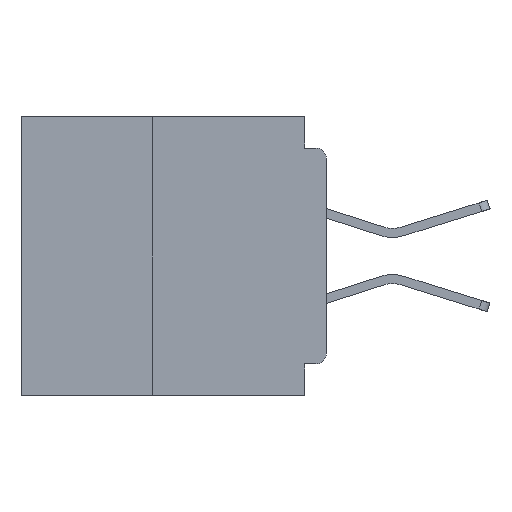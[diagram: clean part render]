
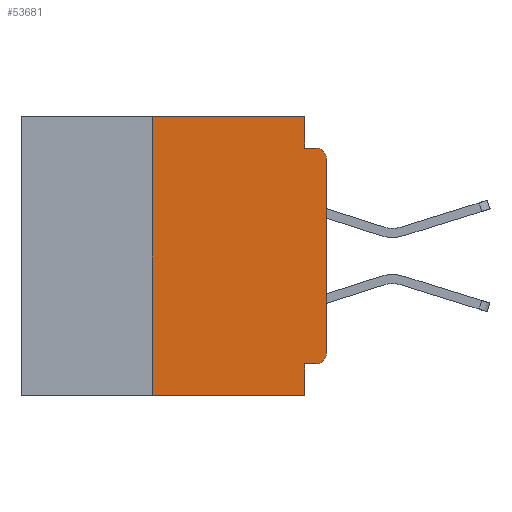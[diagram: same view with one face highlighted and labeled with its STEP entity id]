
A CAD part, left-side view. The second image highlights one B-rep face of the part: STEP entity #53681.
In plain terms, the highlighted planar face has unit normal (-1, 0, 0).
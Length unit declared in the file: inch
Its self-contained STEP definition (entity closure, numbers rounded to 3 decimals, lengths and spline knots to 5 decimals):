
#747 = ORIENTED_EDGE ( 'NONE', *, *, #26089, .T. ) ;
#2071 = CIRCLE ( 'NONE', #11565, 0.015 ) ;
#2143 = ORIENTED_EDGE ( 'NONE', *, *, #19989, .F. ) ;
#2310 = EDGE_CURVE ( 'NONE', #57556, #36472, #18998, .T. ) ;
#2334 = CARTESIAN_POINT ( 'NONE',  ( 0., 0., -0.06 ) ) ;
#3139 = CARTESIAN_POINT ( 'NONE',  ( 0., 0.015, -0.34 ) ) ;
#3239 = VERTEX_POINT ( 'NONE', #44509 ) ;
#3840 = CARTESIAN_POINT ( 'NONE',  ( 0., 0., -0.355 ) ) ;
#3991 = VERTEX_POINT ( 'NONE', #36102 ) ;
#4063 = CARTESIAN_POINT ( 'NONE',  ( 0., 0.015, -0.06 ) ) ;
#4863 = VECTOR ( 'NONE', #22770, 39.37008 ) ;
#5577 = DIRECTION ( 'NONE',  ( 1., 0., 0. ) ) ;
#5811 = DIRECTION ( 'NONE',  ( 0., 0., -1. ) ) ;
#6297 = EDGE_CURVE ( 'NONE', #9676, #44145, #27375, .T. ) ;
#6506 = VERTEX_POINT ( 'NONE', #19624 ) ;
#7970 = DIRECTION ( 'NONE',  ( 0., 0., -1. ) ) ;
#8627 = CARTESIAN_POINT ( 'NONE',  ( 0., 0.015, -0.355 ) ) ;
#8841 = ORIENTED_EDGE ( 'NONE', *, *, #52697, .T. ) ;
#8894 = DIRECTION ( 'NONE',  ( 0., 0., -1. ) ) ;
#9263 = VECTOR ( 'NONE', #47070, 39.37008 ) ;
#9492 = VERTEX_POINT ( 'NONE', #2334 ) ;
#9676 = VERTEX_POINT ( 'NONE', #8627 ) ;
#10426 = ORIENTED_EDGE ( 'NONE', *, *, #38977, .F. ) ;
#10775 = LINE ( 'NONE', #42381, #9263 ) ;
#11336 = AXIS2_PLACEMENT_3D ( 'NONE', #4063, #37016, #8894 ) ;
#11565 = AXIS2_PLACEMENT_3D ( 'NONE', #3139, #36144, #7970 ) ;
#13923 = CARTESIAN_POINT ( 'NONE',  ( 0., 0., -0.34 ) ) ;
#14379 = CARTESIAN_POINT ( 'NONE',  ( 0., 0.031, 0. ) ) ;
#16612 = ORIENTED_EDGE ( 'NONE', *, *, #2310, .F. ) ;
#17891 = EDGE_LOOP ( 'NONE', ( #35993, #747, #55566, #55245, #16612, #2143, #58417, #10426, #19688, #8841 ) ) ;
#18208 = VECTOR ( 'NONE', #31774, 39.37008 ) ;
#18998 = LINE ( 'NONE', #26591, #4863 ) ;
#19624 = CARTESIAN_POINT ( 'NONE',  ( 0., 0.25, -0.4 ) ) ;
#19688 = ORIENTED_EDGE ( 'NONE', *, *, #6297, .F. ) ;
#19908 = VECTOR ( 'NONE', #5811, 39.37008 ) ;
#19989 = EDGE_CURVE ( 'NONE', #6506, #57556, #46545, .T. ) ;
#22770 = DIRECTION ( 'NONE',  ( 0., -1., 0. ) ) ;
#23812 = EDGE_CURVE ( 'NONE', #36472, #3239, #44703, .T. ) ;
#25029 = FACE_OUTER_BOUND ( 'NONE', #17891, .T. ) ;
#26089 = EDGE_CURVE ( 'NONE', #9492, #35049, #53801, .T. ) ;
#26181 = CARTESIAN_POINT ( 'NONE',  ( 0., 0.015, -0.045 ) ) ;
#26591 = CARTESIAN_POINT ( 'NONE',  ( 0., 0.437, 0. ) ) ;
#27087 = CARTESIAN_POINT ( 'NONE',  ( 0., 0.25, 0. ) ) ;
#27115 = CARTESIAN_POINT ( 'NONE',  ( 0., 0.031, -0.4 ) ) ;
#27375 = LINE ( 'NONE', #3840, #38195 ) ;
#30188 = VECTOR ( 'NONE', #50889, 39.37008 ) ;
#31169 = EDGE_CURVE ( 'NONE', #3239, #35049, #42478, .T. ) ;
#31774 = DIRECTION ( 'NONE',  ( 0., 0., -1. ) ) ;
#32280 = EDGE_CURVE ( 'NONE', #6506, #3991, #52225, .T. ) ;
#33648 = CARTESIAN_POINT ( 'NONE',  ( 0., 0.031, -0.355 ) ) ;
#33813 = PLANE ( 'NONE',  #59173 ) ;
#35049 = VERTEX_POINT ( 'NONE', #26181 ) ;
#35993 = ORIENTED_EDGE ( 'NONE', *, *, #36467, .T. ) ;
#36102 = CARTESIAN_POINT ( 'NONE',  ( 0., 0.031, -0.4 ) ) ;
#36144 = DIRECTION ( 'NONE',  ( -1., 0., 0. ) ) ;
#36467 = EDGE_CURVE ( 'NONE', #36879, #9492, #10775, .T. ) ;
#36472 = VERTEX_POINT ( 'NONE', #14379 ) ;
#36879 = VERTEX_POINT ( 'NONE', #13923 ) ;
#37016 = DIRECTION ( 'NONE',  ( -1., 0., 0. ) ) ;
#38195 = VECTOR ( 'NONE', #41443, 39.37008 ) ;
#38427 = DIRECTION ( 'NONE',  ( 0., 0., -1. ) ) ;
#38638 = CARTESIAN_POINT ( 'NONE',  ( 0., 0.031, 0. ) ) ;
#38977 = EDGE_CURVE ( 'NONE', #44145, #3991, #55328, .T. ) ;
#39874 = VECTOR ( 'NONE', #40391, 39.37008 ) ;
#40391 = DIRECTION ( 'NONE',  ( 0., -1., 0. ) ) ;
#41350 = CARTESIAN_POINT ( 'NONE',  ( 0., 0.25, -0.4 ) ) ;
#41443 = DIRECTION ( 'NONE',  ( 0., 1., 0. ) ) ;
#42381 = CARTESIAN_POINT ( 'NONE',  ( 0., 0., 0. ) ) ;
#42478 = LINE ( 'NONE', #59915, #30188 ) ;
#44145 = VERTEX_POINT ( 'NONE', #33648 ) ;
#44509 = CARTESIAN_POINT ( 'NONE',  ( 0., 0.031, -0.045 ) ) ;
#44703 = LINE ( 'NONE', #38638, #19908 ) ;
#46064 = DIRECTION ( 'NONE',  ( 0., 0., 1. ) ) ;
#46545 = LINE ( 'NONE', #41350, #47997 ) ;
#47070 = DIRECTION ( 'NONE',  ( 0., 0., 1. ) ) ;
#47997 = VECTOR ( 'NONE', #46064, 39.37008 ) ;
#50889 = DIRECTION ( 'NONE',  ( 0., -1., 0. ) ) ;
#52225 = LINE ( 'NONE', #54374, #39874 ) ;
#52240 = CARTESIAN_POINT ( 'NONE',  ( 0., 0.437, 0. ) ) ;
#52697 = EDGE_CURVE ( 'NONE', #9676, #36879, #2071, .T. ) ;
#53681 = ADVANCED_FACE ( 'NONE', ( #25029 ), #33813, .F. ) ;
#53801 = CIRCLE ( 'NONE', #11336, 0.015 ) ;
#54374 = CARTESIAN_POINT ( 'NONE',  ( 0., 0.437, -0.4 ) ) ;
#55245 = ORIENTED_EDGE ( 'NONE', *, *, #23812, .F. ) ;
#55328 = LINE ( 'NONE', #27115, #18208 ) ;
#55566 = ORIENTED_EDGE ( 'NONE', *, *, #31169, .F. ) ;
#57556 = VERTEX_POINT ( 'NONE', #27087 ) ;
#58417 = ORIENTED_EDGE ( 'NONE', *, *, #32280, .T. ) ;
#59173 = AXIS2_PLACEMENT_3D ( 'NONE', #52240, #5577, #38427 ) ;
#59915 = CARTESIAN_POINT ( 'NONE',  ( 0., 0., -0.045 ) ) ;
